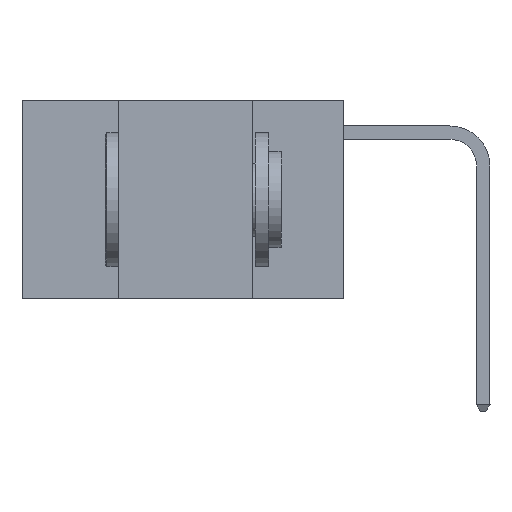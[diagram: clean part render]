
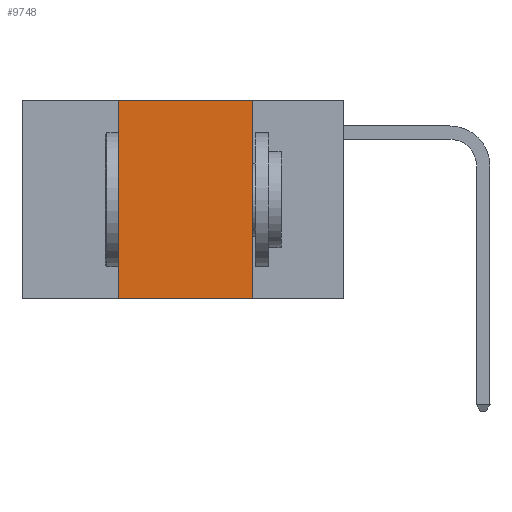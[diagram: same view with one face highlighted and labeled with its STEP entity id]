
A CAD part, left-side view. The second image highlights one B-rep face of the part: STEP entity #9748.
In plain terms, the highlighted planar face has unit normal (-1, 0, 0).
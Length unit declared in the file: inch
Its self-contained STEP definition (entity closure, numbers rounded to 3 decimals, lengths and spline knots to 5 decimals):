
#191 = ORIENTED_EDGE ( 'NONE', *, *, #23493, .F. ) ;
#238 = VERTEX_POINT ( 'NONE', #3363 ) ;
#454 = CARTESIAN_POINT ( 'NONE',  ( 0., 0.17, -0.37 ) ) ;
#622 = ORIENTED_EDGE ( 'NONE', *, *, #26294, .F. ) ;
#1400 = CARTESIAN_POINT ( 'NONE',  ( 0., 0.17, 0. ) ) ;
#1819 = DIRECTION ( 'NONE',  ( 0., 0., -1. ) ) ;
#2944 = DIRECTION ( 'NONE',  ( 0., -1., 0. ) ) ;
#3159 = LINE ( 'NONE', #9572, #16634 ) ;
#3363 = CARTESIAN_POINT ( 'NONE',  ( 0., 0.42, -0.37 ) ) ;
#3376 = CARTESIAN_POINT ( 'NONE',  ( 0., 0.6, 0. ) ) ;
#3887 = CARTESIAN_POINT ( 'NONE',  ( 0., 0.17, 0. ) ) ;
#4958 = VERTEX_POINT ( 'NONE', #454 ) ;
#6296 = VERTEX_POINT ( 'NONE', #1400 ) ;
#6646 = VECTOR ( 'NONE', #18694, 39.37008 ) ;
#7129 = AXIS2_PLACEMENT_3D ( 'NONE', #23614, #17301, #1819 ) ;
#7611 = LINE ( 'NONE', #3376, #17511 ) ;
#9572 = CARTESIAN_POINT ( 'NONE',  ( 0., 0.42, 0. ) ) ;
#9748 = ADVANCED_FACE ( 'NONE', ( #15268 ), #17017, .F. ) ;
#11260 = ORIENTED_EDGE ( 'NONE', *, *, #16329, .T. ) ;
#11683 = CARTESIAN_POINT ( 'NONE',  ( 0., 0.6, -0.37 ) ) ;
#13880 = LINE ( 'NONE', #11683, #6646 ) ;
#15068 = VECTOR ( 'NONE', #19516, 39.37008 ) ;
#15268 = FACE_OUTER_BOUND ( 'NONE', #25099, .T. ) ;
#16329 = EDGE_CURVE ( 'NONE', #238, #4958, #13880, .T. ) ;
#16634 = VECTOR ( 'NONE', #27682, 39.37008 ) ;
#16853 = EDGE_CURVE ( 'NONE', #6296, #4958, #19095, .T. ) ;
#17017 = PLANE ( 'NONE',  #7129 ) ;
#17301 = DIRECTION ( 'NONE',  ( 1., 0., 0. ) ) ;
#17511 = VECTOR ( 'NONE', #2944, 39.37008 ) ;
#18694 = DIRECTION ( 'NONE',  ( 0., -1., 0. ) ) ;
#19095 = LINE ( 'NONE', #3887, #15068 ) ;
#19516 = DIRECTION ( 'NONE',  ( 0., 0., -1. ) ) ;
#21079 = CARTESIAN_POINT ( 'NONE',  ( 0., 0.42, 0. ) ) ;
#21288 = ORIENTED_EDGE ( 'NONE', *, *, #16853, .F. ) ;
#23493 = EDGE_CURVE ( 'NONE', #28060, #6296, #7611, .T. ) ;
#23614 = CARTESIAN_POINT ( 'NONE',  ( 0., 0.6, 0. ) ) ;
#25099 = EDGE_LOOP ( 'NONE', ( #21288, #191, #622, #11260 ) ) ;
#26294 = EDGE_CURVE ( 'NONE', #238, #28060, #3159, .T. ) ;
#27682 = DIRECTION ( 'NONE',  ( 0., 0., 1. ) ) ;
#28060 = VERTEX_POINT ( 'NONE', #21079 ) ;
